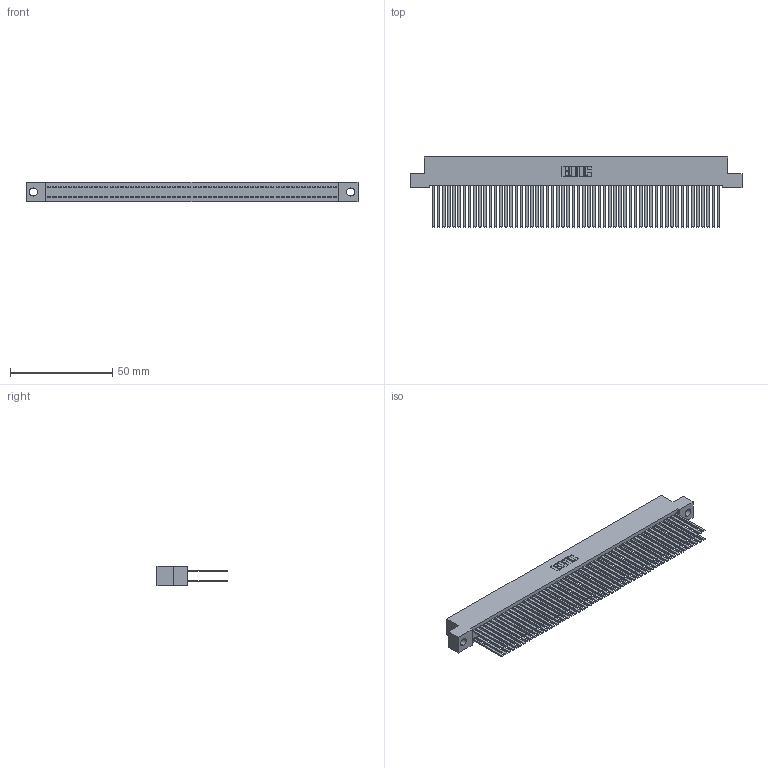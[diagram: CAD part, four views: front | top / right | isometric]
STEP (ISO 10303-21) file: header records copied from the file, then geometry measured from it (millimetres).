
FILE_DESCRIPTION (( 'STEP AP203' ), '1' );
FILE_NAME ('392-112-544-204.STEP', '2018-08-18T22:38:40', ( '' ), ( '' ), 'SwSTEP 2.0', 'SolidWorks 2016', '' );
FILE_SCHEMA (( 'CONFIG_CONTROL_DESIGN' ));
Length unit declared in the file: inch
Products named in the file (3): 342 Part_.156 TH; 345-292-001_345-293-144; 392-112-544-204
Assembly tree (113 placements, depth 2):
  392-112-544-204
    342 Part_.156 TH
    345-292-001_345-293-144  x112
Bounding box: 162.56 x 34.3 x 9.4 mm (x, y, z)
Volume: 16155.3 mm3; surface area: 30813.9 mm2
Topology: 113 solids, 113 shells, 5262 faces, 15643 edges, 10278 vertices
Faces by surface type: plane 3650, cylinder 1612
Entity records: 33903 total; most frequent: CARTESIAN_POINT 5598, ORIENTED_EDGE 5534, DIRECTION 4755, EDGE_CURVE 2767, VECTOR 2643, LINE 2643, VERTEX_POINT 1842, AXIS2_PLACEMENT_3D 1056
